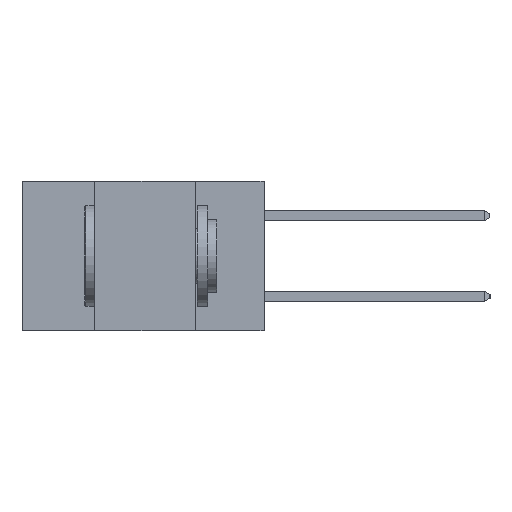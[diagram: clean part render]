
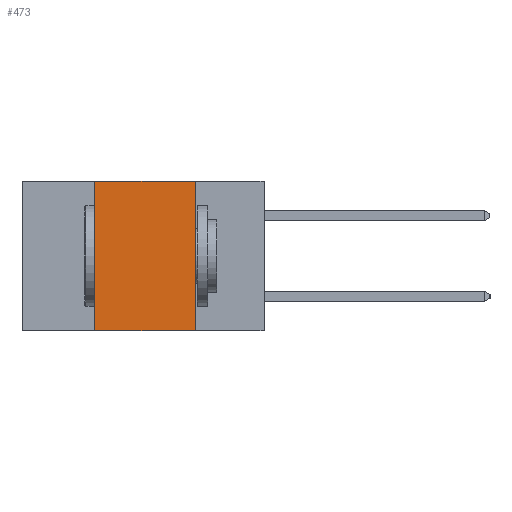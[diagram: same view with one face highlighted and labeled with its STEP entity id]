
A CAD part, left-side view. The second image highlights one B-rep face of the part: STEP entity #473.
In plain terms, the highlighted planar face has unit normal (-1, 0, 0).
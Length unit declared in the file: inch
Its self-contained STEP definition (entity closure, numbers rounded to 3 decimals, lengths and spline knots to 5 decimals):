
#158 = DIRECTION ( 'NONE',  ( 0., -1., 0. ) ) ;
#473 = ADVANCED_FACE ( 'NONE', ( #8757 ), #7034, .F. ) ;
#1068 = CARTESIAN_POINT ( 'NONE',  ( 0., 0.42, 0. ) ) ;
#1091 = LINE ( 'NONE', #3338, #8308 ) ;
#1206 = ORIENTED_EDGE ( 'NONE', *, *, #11975, .F. ) ;
#1663 = DIRECTION ( 'NONE',  ( 1., 0., 0. ) ) ;
#1848 = VERTEX_POINT ( 'NONE', #5257 ) ;
#1896 = DIRECTION ( 'NONE',  ( 0., 0., -1. ) ) ;
#2173 = ORIENTED_EDGE ( 'NONE', *, *, #8544, .F. ) ;
#2489 = ORIENTED_EDGE ( 'NONE', *, *, #7301, .T. ) ;
#2558 = DIRECTION ( 'NONE',  ( 0., 0., 1. ) ) ;
#3338 = CARTESIAN_POINT ( 'NONE',  ( 0., 0.6, 0. ) ) ;
#3660 = CARTESIAN_POINT ( 'NONE',  ( 0., 0.17, -0.37 ) ) ;
#4008 = LINE ( 'NONE', #10223, #8813 ) ;
#4275 = CARTESIAN_POINT ( 'NONE',  ( 0., 0.6, -0.37 ) ) ;
#4378 = VERTEX_POINT ( 'NONE', #12322 ) ;
#4686 = VECTOR ( 'NONE', #9414, 39.37008 ) ;
#4798 = EDGE_CURVE ( 'NONE', #10866, #10939, #4008, .T. ) ;
#5257 = CARTESIAN_POINT ( 'NONE',  ( 0., 0.17, 0. ) ) ;
#6024 = EDGE_LOOP ( 'NONE', ( #1206, #2173, #7381, #2489 ) ) ;
#6163 = CARTESIAN_POINT ( 'NONE',  ( 0., 0.6, 0. ) ) ;
#7034 = PLANE ( 'NONE',  #7137 ) ;
#7137 = AXIS2_PLACEMENT_3D ( 'NONE', #6163, #1663, #1896 ) ;
#7301 = EDGE_CURVE ( 'NONE', #10866, #4378, #11566, .T. ) ;
#7381 = ORIENTED_EDGE ( 'NONE', *, *, #4798, .F. ) ;
#8308 = VECTOR ( 'NONE', #158, 39.37008 ) ;
#8544 = EDGE_CURVE ( 'NONE', #10939, #1848, #1091, .T. ) ;
#8757 = FACE_OUTER_BOUND ( 'NONE', #6024, .T. ) ;
#8813 = VECTOR ( 'NONE', #2558, 39.37008 ) ;
#9414 = DIRECTION ( 'NONE',  ( 0., 0., -1. ) ) ;
#9485 = VECTOR ( 'NONE', #11722, 39.37008 ) ;
#10034 = LINE ( 'NONE', #3660, #4686 ) ;
#10223 = CARTESIAN_POINT ( 'NONE',  ( 0., 0.42, -0.37 ) ) ;
#10650 = CARTESIAN_POINT ( 'NONE',  ( 0., 0.42, -0.37 ) ) ;
#10866 = VERTEX_POINT ( 'NONE', #10650 ) ;
#10939 = VERTEX_POINT ( 'NONE', #1068 ) ;
#11566 = LINE ( 'NONE', #4275, #9485 ) ;
#11722 = DIRECTION ( 'NONE',  ( 0., -1., 0. ) ) ;
#11975 = EDGE_CURVE ( 'NONE', #1848, #4378, #10034, .T. ) ;
#12322 = CARTESIAN_POINT ( 'NONE',  ( 0., 0.17, -0.37 ) ) ;
